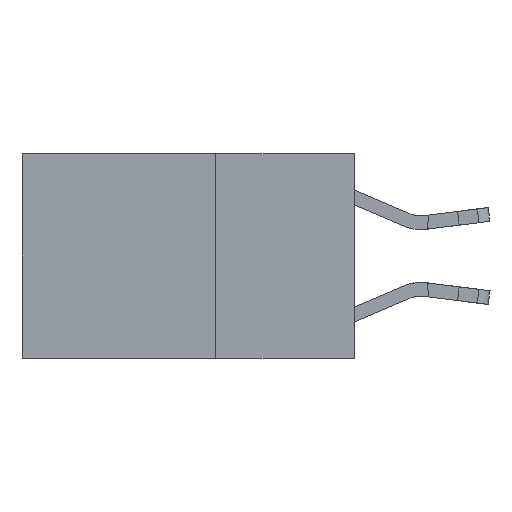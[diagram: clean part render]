
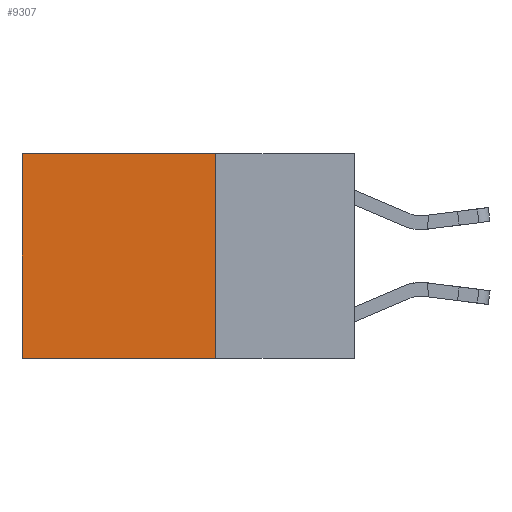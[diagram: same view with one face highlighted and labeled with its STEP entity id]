
A CAD part, left-side view. The second image highlights one B-rep face of the part: STEP entity #9307.
In plain terms, the highlighted planar face has unit normal (-1, 0, 0).
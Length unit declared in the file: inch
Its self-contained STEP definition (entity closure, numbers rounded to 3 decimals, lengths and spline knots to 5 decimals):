
#221 = VECTOR ( 'NONE', #22599, 39.37008 ) ;
#464 = VERTEX_POINT ( 'NONE', #2199 ) ;
#863 = ORIENTED_EDGE ( 'NONE', *, *, #19279, .F. ) ;
#1517 = EDGE_CURVE ( 'NONE', #8644, #464, #19519, .T. ) ;
#2199 = CARTESIAN_POINT ( 'NONE',  ( 0.2625, 0.6, -0.37 ) ) ;
#2753 = CARTESIAN_POINT ( 'NONE',  ( 0.2625, 0.25, 0. ) ) ;
#3445 = VERTEX_POINT ( 'NONE', #18940 ) ;
#4462 = LINE ( 'NONE', #23177, #5086 ) ;
#4739 = DIRECTION ( 'NONE',  ( 0., 0., -1. ) ) ;
#5086 = VECTOR ( 'NONE', #15562, 39.37008 ) ;
#5555 = LINE ( 'NONE', #9128, #221 ) ;
#5981 = EDGE_LOOP ( 'NONE', ( #6520, #14487, #863, #9093 ) ) ;
#6520 = ORIENTED_EDGE ( 'NONE', *, *, #14878, .T. ) ;
#6977 = CARTESIAN_POINT ( 'NONE',  ( 0.2625, 0.6, 0. ) ) ;
#7646 = CARTESIAN_POINT ( 'NONE',  ( 0.2625, 0.25, -0.37 ) ) ;
#8237 = PLANE ( 'NONE',  #9742 ) ;
#8417 = VECTOR ( 'NONE', #4739, 39.37008 ) ;
#8644 = VERTEX_POINT ( 'NONE', #7646 ) ;
#9093 = ORIENTED_EDGE ( 'NONE', *, *, #23872, .T. ) ;
#9128 = CARTESIAN_POINT ( 'NONE',  ( 0.2625, 0.6, 0. ) ) ;
#9307 = ADVANCED_FACE ( 'NONE', ( #14491 ), #8237, .F. ) ;
#9742 = AXIS2_PLACEMENT_3D ( 'NONE', #17899, #21732, #10184 ) ;
#10184 = DIRECTION ( 'NONE',  ( 0., 0., -1. ) ) ;
#14487 = ORIENTED_EDGE ( 'NONE', *, *, #1517, .F. ) ;
#14491 = FACE_OUTER_BOUND ( 'NONE', #5981, .T. ) ;
#14693 = CARTESIAN_POINT ( 'NONE',  ( 0.2625, 0.25, -0.37 ) ) ;
#14878 = EDGE_CURVE ( 'NONE', #19686, #464, #5555, .T. ) ;
#15562 = DIRECTION ( 'NONE',  ( 0., 1., 0. ) ) ;
#17877 = DIRECTION ( 'NONE',  ( 0., 1., 0. ) ) ;
#17899 = CARTESIAN_POINT ( 'NONE',  ( 0.2625, 0.25, 0. ) ) ;
#18739 = LINE ( 'NONE', #2753, #8417 ) ;
#18921 = VECTOR ( 'NONE', #17877, 39.37008 ) ;
#18940 = CARTESIAN_POINT ( 'NONE',  ( 0.2625, 0.25, 0. ) ) ;
#19279 = EDGE_CURVE ( 'NONE', #3445, #8644, #18739, .T. ) ;
#19519 = LINE ( 'NONE', #14693, #18921 ) ;
#19686 = VERTEX_POINT ( 'NONE', #6977 ) ;
#21732 = DIRECTION ( 'NONE',  ( 1., 0., 0. ) ) ;
#22599 = DIRECTION ( 'NONE',  ( 0., 0., -1. ) ) ;
#23177 = CARTESIAN_POINT ( 'NONE',  ( 0.2625, 0.25, 0. ) ) ;
#23872 = EDGE_CURVE ( 'NONE', #3445, #19686, #4462, .T. ) ;
